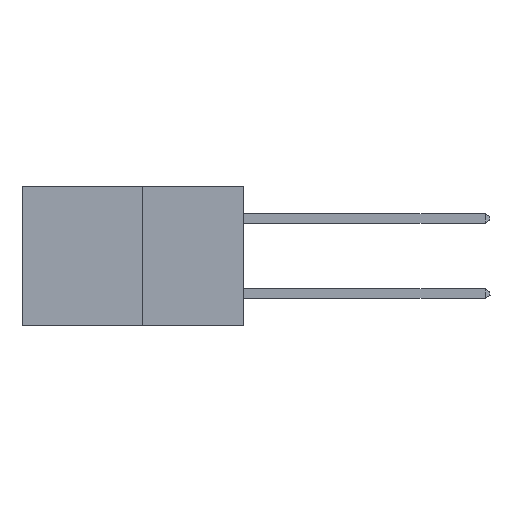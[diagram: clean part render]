
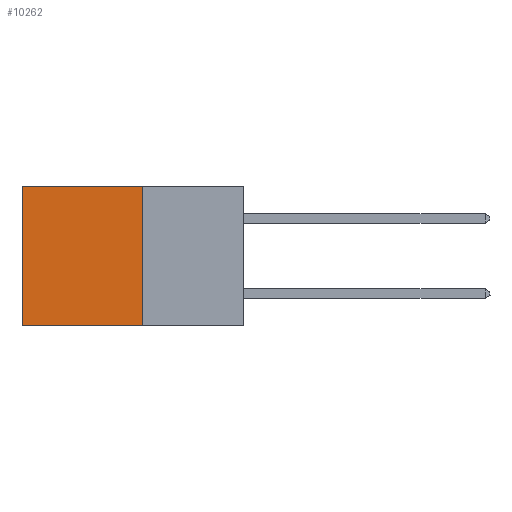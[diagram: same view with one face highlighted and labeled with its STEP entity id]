
A CAD part, left-side view. The second image highlights one B-rep face of the part: STEP entity #10262.
In plain terms, the highlighted planar face has unit normal (-1, 0, 0).
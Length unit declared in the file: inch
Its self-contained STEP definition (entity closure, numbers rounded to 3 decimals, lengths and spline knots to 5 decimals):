
#376 = CARTESIAN_POINT ( 'NONE',  ( 0.277, 0.27, -0.37 ) ) ;
#449 = CARTESIAN_POINT ( 'NONE',  ( 0.277, 0.27, 0. ) ) ;
#493 = CARTESIAN_POINT ( 'NONE',  ( 0.277, 0.59, 0. ) ) ;
#977 = CARTESIAN_POINT ( 'NONE',  ( 0.277, 0.27, -0.37 ) ) ;
#2789 = VERTEX_POINT ( 'NONE', #7580 ) ;
#3019 = VECTOR ( 'NONE', #3072, 39.37008 ) ;
#3035 = LINE ( 'NONE', #977, #16812 ) ;
#3072 = DIRECTION ( 'NONE',  ( 0., 0., -1. ) ) ;
#3433 = LINE ( 'NONE', #376, #3019 ) ;
#4355 = FACE_OUTER_BOUND ( 'NONE', #14400, .T. ) ;
#6303 = CARTESIAN_POINT ( 'NONE',  ( 0.277, 0.27, -0.37 ) ) ;
#6862 = DIRECTION ( 'NONE',  ( 0., 0., -1. ) ) ;
#7520 = ORIENTED_EDGE ( 'NONE', *, *, #15454, .F. ) ;
#7532 = CARTESIAN_POINT ( 'NONE',  ( 0.277, 0.59, -0.37 ) ) ;
#7580 = CARTESIAN_POINT ( 'NONE',  ( 0.277, 0.27, -0.37 ) ) ;
#7646 = DIRECTION ( 'NONE',  ( 1., 0., 0. ) ) ;
#8048 = ORIENTED_EDGE ( 'NONE', *, *, #16082, .T. ) ;
#8472 = DIRECTION ( 'NONE',  ( 0., 1., 0. ) ) ;
#8999 = EDGE_CURVE ( 'NONE', #16151, #9595, #14598, .T. ) ;
#9379 = ORIENTED_EDGE ( 'NONE', *, *, #8999, .T. ) ;
#9595 = VERTEX_POINT ( 'NONE', #493 ) ;
#9911 = LINE ( 'NONE', #14821, #14257 ) ;
#10262 = ADVANCED_FACE ( 'NONE', ( #4355 ), #14260, .F. ) ;
#11855 = ORIENTED_EDGE ( 'NONE', *, *, #15876, .F. ) ;
#13832 = VERTEX_POINT ( 'NONE', #7532 ) ;
#14257 = VECTOR ( 'NONE', #6862, 39.37008 ) ;
#14260 = PLANE ( 'NONE',  #14370 ) ;
#14370 = AXIS2_PLACEMENT_3D ( 'NONE', #6303, #7646, #16965 ) ;
#14400 = EDGE_LOOP ( 'NONE', ( #8048, #7520, #11855, #9379 ) ) ;
#14598 = LINE ( 'NONE', #449, #16914 ) ;
#14821 = CARTESIAN_POINT ( 'NONE',  ( 0.277, 0.59, -0.37 ) ) ;
#14923 = CARTESIAN_POINT ( 'NONE',  ( 0.277, 0.27, 0. ) ) ;
#15454 = EDGE_CURVE ( 'NONE', #2789, #13832, #3035, .T. ) ;
#15615 = DIRECTION ( 'NONE',  ( 0., 1., 0. ) ) ;
#15876 = EDGE_CURVE ( 'NONE', #16151, #2789, #3433, .T. ) ;
#16082 = EDGE_CURVE ( 'NONE', #9595, #13832, #9911, .T. ) ;
#16151 = VERTEX_POINT ( 'NONE', #14923 ) ;
#16812 = VECTOR ( 'NONE', #15615, 39.37008 ) ;
#16914 = VECTOR ( 'NONE', #8472, 39.37008 ) ;
#16965 = DIRECTION ( 'NONE',  ( 0., 0., -1. ) ) ;
